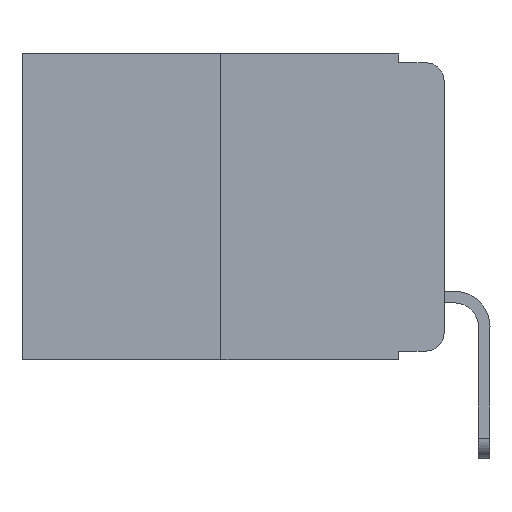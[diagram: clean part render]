
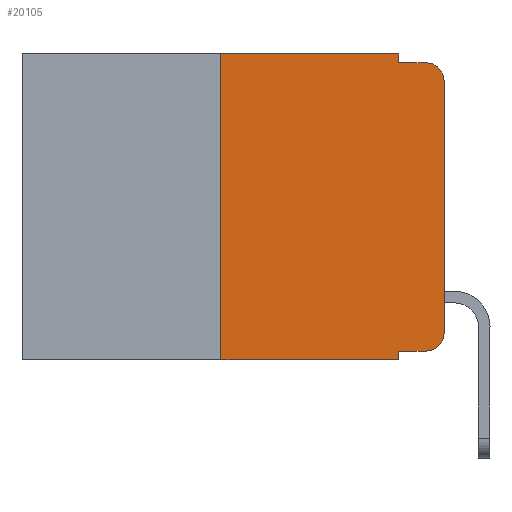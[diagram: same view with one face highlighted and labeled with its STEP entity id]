
A CAD part, left-side view. The second image highlights one B-rep face of the part: STEP entity #20105.
In plain terms, the highlighted planar face has unit normal (-1, 0, 0).
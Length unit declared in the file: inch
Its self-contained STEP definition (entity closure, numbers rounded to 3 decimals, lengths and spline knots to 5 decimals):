
#202 = DIRECTION ( 'NONE',  ( -1., 0., 0. ) ) ;
#730 = EDGE_CURVE ( 'NONE', #18435, #9059, #1698, .T. ) ;
#789 = VERTEX_POINT ( 'NONE', #9981 ) ;
#1306 = CARTESIAN_POINT ( 'NONE',  ( 0., 0., 0. ) ) ;
#1607 = CARTESIAN_POINT ( 'NONE',  ( 0., 0.473, 0. ) ) ;
#1698 = LINE ( 'NONE', #8123, #12717 ) ;
#1926 = AXIS2_PLACEMENT_3D ( 'NONE', #19688, #2204, #18095 ) ;
#1955 = CARTESIAN_POINT ( 'NONE',  ( 0., 0.25, 0. ) ) ;
#1979 = VERTEX_POINT ( 'NONE', #11132 ) ;
#2204 = DIRECTION ( 'NONE',  ( -1., 0., 0. ) ) ;
#2253 = CARTESIAN_POINT ( 'NONE',  ( 0., 0.25, 0. ) ) ;
#3009 = VECTOR ( 'NONE', #9353, 39.37008 ) ;
#3258 = ORIENTED_EDGE ( 'NONE', *, *, #730, .T. ) ;
#3769 = ORIENTED_EDGE ( 'NONE', *, *, #8997, .F. ) ;
#4245 = CARTESIAN_POINT ( 'NONE',  ( 0., 0.051, -0.343 ) ) ;
#4615 = ORIENTED_EDGE ( 'NONE', *, *, #13324, .T. ) ;
#4905 = DIRECTION ( 'NONE',  ( 0., 0., -1. ) ) ;
#4937 = ORIENTED_EDGE ( 'NONE', *, *, #5590, .T. ) ;
#5583 = LINE ( 'NONE', #15556, #12368 ) ;
#5590 = EDGE_CURVE ( 'NONE', #13989, #19216, #8493, .T. ) ;
#5625 = CARTESIAN_POINT ( 'NONE',  ( 0., 0.02, -0.01 ) ) ;
#6246 = VERTEX_POINT ( 'NONE', #18704 ) ;
#6597 = CARTESIAN_POINT ( 'NONE',  ( 0., 0.02, -0.313 ) ) ;
#6877 = CARTESIAN_POINT ( 'NONE',  ( 0., 0.051, -0.333 ) ) ;
#7036 = EDGE_CURVE ( 'NONE', #9059, #14186, #18726, .T. ) ;
#7490 = VECTOR ( 'NONE', #14617, 39.37008 ) ;
#7915 = EDGE_LOOP ( 'NONE', ( #4615, #4937, #13995, #12852, #15802, #3769, #18164, #10305, #3258, #13696 ) ) ;
#7990 = AXIS2_PLACEMENT_3D ( 'NONE', #6597, #202, #4905 ) ;
#8123 = CARTESIAN_POINT ( 'NONE',  ( 0., 0.051, -0.333 ) ) ;
#8183 = CARTESIAN_POINT ( 'NONE',  ( 0., 0.051, 0. ) ) ;
#8493 = CIRCLE ( 'NONE', #1926, 0.02 ) ;
#8586 = PLANE ( 'NONE',  #11294 ) ;
#8614 = CARTESIAN_POINT ( 'NONE',  ( 0., 0., -0.313 ) ) ;
#8997 = EDGE_CURVE ( 'NONE', #789, #14108, #18288, .T. ) ;
#9059 = VERTEX_POINT ( 'NONE', #17975 ) ;
#9353 = DIRECTION ( 'NONE',  ( 0., 0., 1. ) ) ;
#9981 = CARTESIAN_POINT ( 'NONE',  ( 0., 0.25, -0.343 ) ) ;
#10305 = ORIENTED_EDGE ( 'NONE', *, *, #19323, .F. ) ;
#10586 = LINE ( 'NONE', #11801, #14558 ) ;
#11132 = CARTESIAN_POINT ( 'NONE',  ( 0., 0.051, 0. ) ) ;
#11294 = AXIS2_PLACEMENT_3D ( 'NONE', #11676, #13438, #15009 ) ;
#11676 = CARTESIAN_POINT ( 'NONE',  ( 0., 0.473, 0. ) ) ;
#11687 = EDGE_CURVE ( 'NONE', #14108, #1979, #20598, .T. ) ;
#11744 = LINE ( 'NONE', #8183, #7490 ) ;
#11801 = CARTESIAN_POINT ( 'NONE',  ( 0., 0.051, -0.01 ) ) ;
#12060 = VERTEX_POINT ( 'NONE', #4245 ) ;
#12331 = EDGE_CURVE ( 'NONE', #6246, #19216, #10586, .T. ) ;
#12368 = VECTOR ( 'NONE', #20383, 39.37008 ) ;
#12408 = DIRECTION ( 'NONE',  ( 0., -1., 0. ) ) ;
#12717 = VECTOR ( 'NONE', #17765, 39.37008 ) ;
#12807 = DIRECTION ( 'NONE',  ( 0., -1., 0. ) ) ;
#12852 = ORIENTED_EDGE ( 'NONE', *, *, #15126, .F. ) ;
#13033 = VECTOR ( 'NONE', #17961, 39.37008 ) ;
#13324 = EDGE_CURVE ( 'NONE', #14186, #13989, #17014, .T. ) ;
#13438 = DIRECTION ( 'NONE',  ( 1., 0., 0. ) ) ;
#13696 = ORIENTED_EDGE ( 'NONE', *, *, #7036, .T. ) ;
#13989 = VERTEX_POINT ( 'NONE', #16488 ) ;
#13995 = ORIENTED_EDGE ( 'NONE', *, *, #12331, .F. ) ;
#14108 = VERTEX_POINT ( 'NONE', #2253 ) ;
#14186 = VERTEX_POINT ( 'NONE', #8614 ) ;
#14558 = VECTOR ( 'NONE', #16435, 39.37008 ) ;
#14617 = DIRECTION ( 'NONE',  ( 0., 0., -1. ) ) ;
#14797 = FACE_OUTER_BOUND ( 'NONE', #7915, .T. ) ;
#15009 = DIRECTION ( 'NONE',  ( 0., 0., -1. ) ) ;
#15126 = EDGE_CURVE ( 'NONE', #1979, #6246, #11744, .T. ) ;
#15556 = CARTESIAN_POINT ( 'NONE',  ( 0., 0.051, 0. ) ) ;
#15802 = ORIENTED_EDGE ( 'NONE', *, *, #11687, .F. ) ;
#16435 = DIRECTION ( 'NONE',  ( 0., -1., 0. ) ) ;
#16488 = CARTESIAN_POINT ( 'NONE',  ( 0., 0., -0.03 ) ) ;
#17014 = LINE ( 'NONE', #1306, #3009 ) ;
#17067 = CARTESIAN_POINT ( 'NONE',  ( 0., 0.473, -0.343 ) ) ;
#17594 = VECTOR ( 'NONE', #12807, 39.37008 ) ;
#17765 = DIRECTION ( 'NONE',  ( 0., -1., 0. ) ) ;
#17961 = DIRECTION ( 'NONE',  ( 0., 0., 1. ) ) ;
#17975 = CARTESIAN_POINT ( 'NONE',  ( 0., 0.02, -0.333 ) ) ;
#18078 = VECTOR ( 'NONE', #12408, 39.37008 ) ;
#18095 = DIRECTION ( 'NONE',  ( 0., 0., -1. ) ) ;
#18164 = ORIENTED_EDGE ( 'NONE', *, *, #19893, .T. ) ;
#18288 = LINE ( 'NONE', #1955, #13033 ) ;
#18435 = VERTEX_POINT ( 'NONE', #6877 ) ;
#18704 = CARTESIAN_POINT ( 'NONE',  ( 0., 0.051, -0.01 ) ) ;
#18726 = CIRCLE ( 'NONE', #7990, 0.02 ) ;
#18849 = LINE ( 'NONE', #17067, #18078 ) ;
#19216 = VERTEX_POINT ( 'NONE', #5625 ) ;
#19323 = EDGE_CURVE ( 'NONE', #18435, #12060, #5583, .T. ) ;
#19688 = CARTESIAN_POINT ( 'NONE',  ( 0., 0.02, -0.03 ) ) ;
#19893 = EDGE_CURVE ( 'NONE', #789, #12060, #18849, .T. ) ;
#20105 = ADVANCED_FACE ( 'NONE', ( #14797 ), #8586, .F. ) ;
#20383 = DIRECTION ( 'NONE',  ( 0., 0., -1. ) ) ;
#20598 = LINE ( 'NONE', #1607, #17594 ) ;
